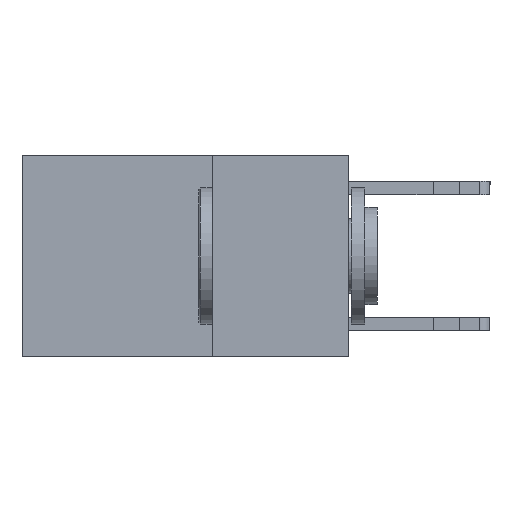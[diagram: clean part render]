
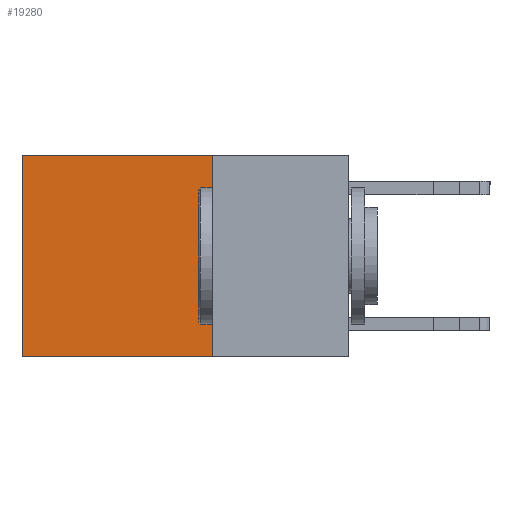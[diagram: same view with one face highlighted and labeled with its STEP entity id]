
A CAD part, left-side view. The second image highlights one B-rep face of the part: STEP entity #19280.
In plain terms, the highlighted planar face has unit normal (-1, 0, 0).
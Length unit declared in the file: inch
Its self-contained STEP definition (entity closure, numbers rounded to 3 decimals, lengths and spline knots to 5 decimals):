
#32 = AXIS2_PLACEMENT_3D ( 'NONE', #23985, #19668, #4904 ) ;
#262 = CARTESIAN_POINT ( 'NONE',  ( 0.2625, 0.6, 0. ) ) ;
#760 = CARTESIAN_POINT ( 'NONE',  ( 0.2625, 0.25, 0. ) ) ;
#793 = ORIENTED_EDGE ( 'NONE', *, *, #26361, .T. ) ;
#862 = LINE ( 'NONE', #9048, #3854 ) ;
#3854 = VECTOR ( 'NONE', #9469, 39.37008 ) ;
#4844 = ORIENTED_EDGE ( 'NONE', *, *, #14716, .F. ) ;
#4904 = DIRECTION ( 'NONE',  ( 0., 0., -1. ) ) ;
#5039 = PLANE ( 'NONE',  #32 ) ;
#5460 = FACE_OUTER_BOUND ( 'NONE', #17339, .T. ) ;
#7035 = VECTOR ( 'NONE', #13402, 39.37008 ) ;
#8567 = CARTESIAN_POINT ( 'NONE',  ( 0.2625, 0.25, 0. ) ) ;
#9048 = CARTESIAN_POINT ( 'NONE',  ( 0.2625, 0.25, 0. ) ) ;
#9202 = ORIENTED_EDGE ( 'NONE', *, *, #16950, .T. ) ;
#9469 = DIRECTION ( 'NONE',  ( 0., 1., 0. ) ) ;
#10824 = VERTEX_POINT ( 'NONE', #262 ) ;
#11644 = CARTESIAN_POINT ( 'NONE',  ( 0.2625, 0.25, -0.37 ) ) ;
#12837 = CARTESIAN_POINT ( 'NONE',  ( 0.2625, 0.6, -0.37 ) ) ;
#13402 = DIRECTION ( 'NONE',  ( 0., 0., -1. ) ) ;
#14697 = VECTOR ( 'NONE', #15274, 39.37008 ) ;
#14716 = EDGE_CURVE ( 'NONE', #23480, #19187, #15243, .T. ) ;
#15243 = LINE ( 'NONE', #760, #7035 ) ;
#15274 = DIRECTION ( 'NONE',  ( 0., 0., -1. ) ) ;
#15879 = VERTEX_POINT ( 'NONE', #12837 ) ;
#16127 = DIRECTION ( 'NONE',  ( 0., 1., 0. ) ) ;
#16950 = EDGE_CURVE ( 'NONE', #10824, #15879, #19182, .T. ) ;
#17093 = CARTESIAN_POINT ( 'NONE',  ( 0.2625, 0.6, 0. ) ) ;
#17339 = EDGE_LOOP ( 'NONE', ( #9202, #26213, #4844, #793 ) ) ;
#17433 = CARTESIAN_POINT ( 'NONE',  ( 0.2625, 0.25, -0.37 ) ) ;
#19182 = LINE ( 'NONE', #17093, #14697 ) ;
#19187 = VERTEX_POINT ( 'NONE', #17433 ) ;
#19280 = ADVANCED_FACE ( 'NONE', ( #5460 ), #5039, .F. ) ;
#19668 = DIRECTION ( 'NONE',  ( 1., 0., 0. ) ) ;
#20160 = VECTOR ( 'NONE', #16127, 39.37008 ) ;
#20465 = LINE ( 'NONE', #11644, #20160 ) ;
#21928 = EDGE_CURVE ( 'NONE', #19187, #15879, #20465, .T. ) ;
#23480 = VERTEX_POINT ( 'NONE', #8567 ) ;
#23985 = CARTESIAN_POINT ( 'NONE',  ( 0.2625, 0.25, 0. ) ) ;
#26213 = ORIENTED_EDGE ( 'NONE', *, *, #21928, .F. ) ;
#26361 = EDGE_CURVE ( 'NONE', #23480, #10824, #862, .T. ) ;
